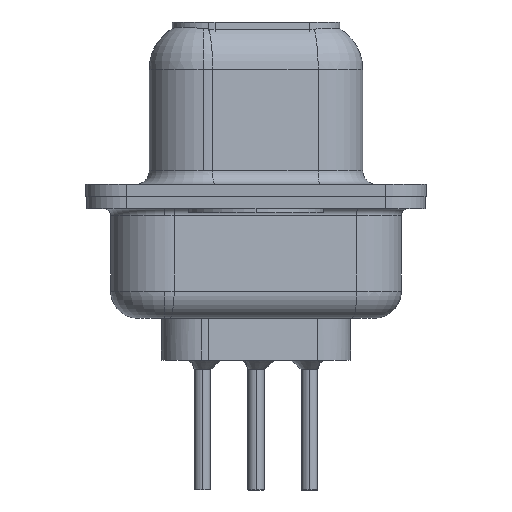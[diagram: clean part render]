
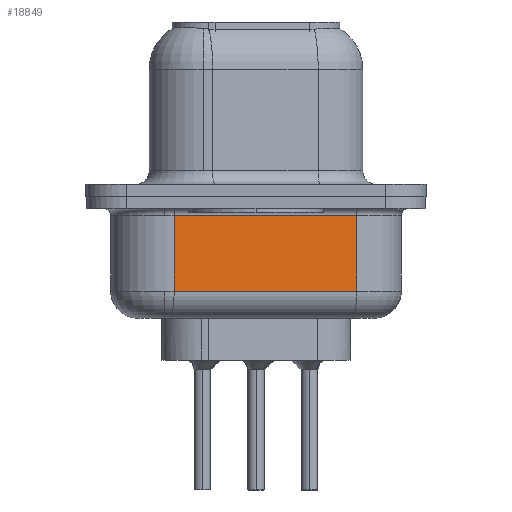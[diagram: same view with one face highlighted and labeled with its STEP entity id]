
A CAD part, left-side view. The second image highlights one B-rep face of the part: STEP entity #18849.
In plain terms, the highlighted planar face has unit normal (-0.985, -0.174, 0).
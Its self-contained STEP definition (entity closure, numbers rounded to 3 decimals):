
#294 = ORIENTED_EDGE ( 'NONE', *, *, #1598, .T. ) ;
#1598 = EDGE_CURVE ( 'NONE', #8955, #14175, #8912, .T. ) ;
#2124 = CARTESIAN_POINT ( 'NONE',  ( 2.925, 3.028, -3.5 ) ) ;
#3164 = DIRECTION ( 'NONE',  ( -0.174, 0.985, 0. ) ) ;
#3415 = ORIENTED_EDGE ( 'NONE', *, *, #9940, .T. ) ;
#4872 = VECTOR ( 'NONE', #9219, 1000. ) ;
#5068 = LINE ( 'NONE', #13391, #9913 ) ;
#5136 = PLANE ( 'NONE',  #18651 ) ;
#5265 = VECTOR ( 'NONE', #16394, 1000. ) ;
#5514 = LINE ( 'NONE', #13223, #4872 ) ;
#6358 = FACE_OUTER_BOUND ( 'NONE', #26342, .T. ) ;
#6560 = LINE ( 'NONE', #26683, #5265 ) ;
#8912 = LINE ( 'NONE', #24768, #19183 ) ;
#8955 = VERTEX_POINT ( 'NONE', #14440 ) ;
#9219 = DIRECTION ( 'NONE',  ( 0., 0., 1. ) ) ;
#9913 = VECTOR ( 'NONE', #3164, 1000. ) ;
#9940 = EDGE_CURVE ( 'NONE', #12212, #8955, #6560, .T. ) ;
#10689 = ORIENTED_EDGE ( 'NONE', *, *, #18262, .T. ) ;
#12212 = VERTEX_POINT ( 'NONE', #2124 ) ;
#12419 = DIRECTION ( 'NONE',  ( 0., 0., 1. ) ) ;
#12477 = EDGE_CURVE ( 'NONE', #12212, #25893, #5514, .T. ) ;
#12531 = CARTESIAN_POINT ( 'NONE',  ( 4.116, -3.722, -0.7 ) ) ;
#13015 = CARTESIAN_POINT ( 'NONE',  ( 2.925, 3.028, -0.7 ) ) ;
#13223 = CARTESIAN_POINT ( 'NONE',  ( 2.925, 3.028, -4.5 ) ) ;
#13360 = DIRECTION ( 'NONE',  ( -0.174, 0.985, 0. ) ) ;
#13391 = CARTESIAN_POINT ( 'NONE',  ( 2.925, 3.028, -0.7 ) ) ;
#14175 = VERTEX_POINT ( 'NONE', #12531 ) ;
#14440 = CARTESIAN_POINT ( 'NONE',  ( 4.116, -3.722, -3.5 ) ) ;
#16394 = DIRECTION ( 'NONE',  ( 0.174, -0.985, 0. ) ) ;
#16686 = ORIENTED_EDGE ( 'NONE', *, *, #12477, .F. ) ;
#18262 = EDGE_CURVE ( 'NONE', #14175, #25893, #5068, .T. ) ;
#18651 = AXIS2_PLACEMENT_3D ( 'NONE', #19494, #25708, #13360 ) ;
#18849 = ADVANCED_FACE ( 'NONE', ( #6358 ), #5136, .F. ) ;
#19183 = VECTOR ( 'NONE', #12419, 1000. ) ;
#19494 = CARTESIAN_POINT ( 'NONE',  ( 2.925, 3.028, -4.5 ) ) ;
#24768 = CARTESIAN_POINT ( 'NONE',  ( 4.116, -3.722, -4.5 ) ) ;
#25708 = DIRECTION ( 'NONE',  ( 0.985, 0.174, 0. ) ) ;
#25893 = VERTEX_POINT ( 'NONE', #13015 ) ;
#26342 = EDGE_LOOP ( 'NONE', ( #16686, #3415, #294, #10689 ) ) ;
#26683 = CARTESIAN_POINT ( 'NONE',  ( 2.925, 3.028, -3.5 ) ) ;
